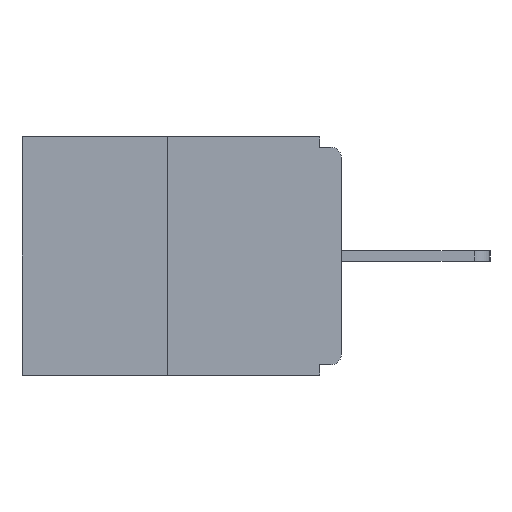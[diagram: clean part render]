
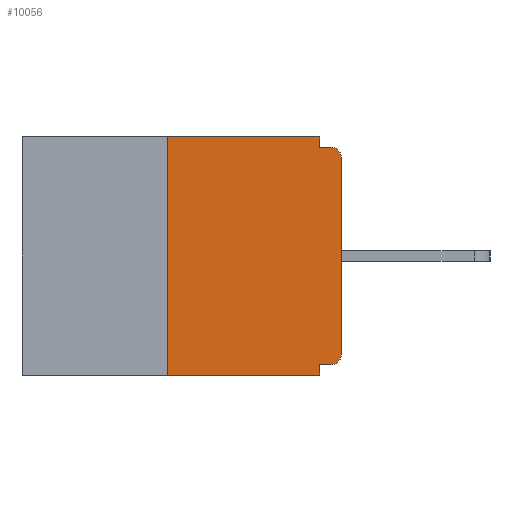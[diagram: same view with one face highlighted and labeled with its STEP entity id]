
A CAD part, left-side view. The second image highlights one B-rep face of the part: STEP entity #10056.
In plain terms, the highlighted planar face has unit normal (-1, 0, 0).
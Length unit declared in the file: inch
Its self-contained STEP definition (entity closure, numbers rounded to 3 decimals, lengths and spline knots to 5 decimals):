
#60 = PLANE ( 'NONE',  #2850 ) ;
#109 = ORIENTED_EDGE ( 'NONE', *, *, #1626, .F. ) ;
#178 = EDGE_LOOP ( 'NONE', ( #8929, #3693, #7737, #2448, #1914, #5647, #10273, #12927, #10424, #109 ) ) ;
#331 = EDGE_CURVE ( 'NONE', #2120, #7161, #4536, .T. ) ;
#432 = LINE ( 'NONE', #6537, #1661 ) ;
#465 = VECTOR ( 'NONE', #6423, 39.37008 ) ;
#608 = VERTEX_POINT ( 'NONE', #2188 ) ;
#852 = DIRECTION ( 'NONE',  ( 0., 0., -1. ) ) ;
#990 = CARTESIAN_POINT ( 'NONE',  ( 0., 0.25, 0. ) ) ;
#1165 = CARTESIAN_POINT ( 'NONE',  ( 0., 0.031, -0.343 ) ) ;
#1224 = VERTEX_POINT ( 'NONE', #3137 ) ;
#1465 = CIRCLE ( 'NONE', #7824, 0.015 ) ;
#1480 = CARTESIAN_POINT ( 'NONE',  ( 0., 0.015, -0.015 ) ) ;
#1555 = CARTESIAN_POINT ( 'NONE',  ( 0., 0., -0.03 ) ) ;
#1626 = EDGE_CURVE ( 'NONE', #608, #5950, #11056, .T. ) ;
#1661 = VECTOR ( 'NONE', #6467, 39.37008 ) ;
#1708 = CARTESIAN_POINT ( 'NONE',  ( 0., 0.015, -0.03 ) ) ;
#1912 = CARTESIAN_POINT ( 'NONE',  ( 0., 0.031, -0.343 ) ) ;
#1914 = ORIENTED_EDGE ( 'NONE', *, *, #2885, .F. ) ;
#2120 = VERTEX_POINT ( 'NONE', #7968 ) ;
#2123 = VECTOR ( 'NONE', #10434, 39.37008 ) ;
#2188 = CARTESIAN_POINT ( 'NONE',  ( 0., 0.031, 0. ) ) ;
#2448 = ORIENTED_EDGE ( 'NONE', *, *, #10078, .F. ) ;
#2670 = EDGE_CURVE ( 'NONE', #10574, #12998, #432, .T. ) ;
#2810 = DIRECTION ( 'NONE',  ( -1., 0., 0. ) ) ;
#2850 = AXIS2_PLACEMENT_3D ( 'NONE', #4093, #8013, #12083 ) ;
#2885 = EDGE_CURVE ( 'NONE', #8611, #1224, #9465, .T. ) ;
#3069 = VECTOR ( 'NONE', #5121, 39.37008 ) ;
#3137 = CARTESIAN_POINT ( 'NONE',  ( 0., 0.031, -0.328 ) ) ;
#3693 = ORIENTED_EDGE ( 'NONE', *, *, #331, .F. ) ;
#3804 = VECTOR ( 'NONE', #7784, 39.37008 ) ;
#4093 = CARTESIAN_POINT ( 'NONE',  ( 0., 0.46, 0. ) ) ;
#4132 = DIRECTION ( 'NONE',  ( 0., 1., 0. ) ) ;
#4360 = CARTESIAN_POINT ( 'NONE',  ( 0., 0.46, 0. ) ) ;
#4429 = LINE ( 'NONE', #4360, #465 ) ;
#4536 = LINE ( 'NONE', #11725, #3804 ) ;
#4790 = VERTEX_POINT ( 'NONE', #1912 ) ;
#5121 = DIRECTION ( 'NONE',  ( 0., 0., -1. ) ) ;
#5245 = EDGE_CURVE ( 'NONE', #12998, #9589, #1465, .T. ) ;
#5251 = CARTESIAN_POINT ( 'NONE',  ( 0., 0., -0.328 ) ) ;
#5427 = CARTESIAN_POINT ( 'NONE',  ( 0., 0., -0.015 ) ) ;
#5647 = ORIENTED_EDGE ( 'NONE', *, *, #12680, .T. ) ;
#5749 = DIRECTION ( 'NONE',  ( -1., 0., 0. ) ) ;
#5808 = CARTESIAN_POINT ( 'NONE',  ( 0., 0.015, -0.313 ) ) ;
#5950 = VERTEX_POINT ( 'NONE', #10644 ) ;
#6162 = EDGE_CURVE ( 'NONE', #5950, #9589, #8215, .T. ) ;
#6244 = VECTOR ( 'NONE', #11150, 39.37008 ) ;
#6365 = VECTOR ( 'NONE', #9177, 39.37008 ) ;
#6423 = DIRECTION ( 'NONE',  ( 0., -1., 0. ) ) ;
#6467 = DIRECTION ( 'NONE',  ( 0., 0., 1. ) ) ;
#6537 = CARTESIAN_POINT ( 'NONE',  ( 0., 0., 0. ) ) ;
#6703 = AXIS2_PLACEMENT_3D ( 'NONE', #5808, #2810, #10951 ) ;
#6748 = EDGE_CURVE ( 'NONE', #2120, #4790, #12362, .T. ) ;
#7029 = LINE ( 'NONE', #1165, #6244 ) ;
#7161 = VERTEX_POINT ( 'NONE', #990 ) ;
#7297 = CARTESIAN_POINT ( 'NONE',  ( 0., 0.46, -0.343 ) ) ;
#7299 = EDGE_CURVE ( 'NONE', #7161, #608, #4429, .T. ) ;
#7737 = ORIENTED_EDGE ( 'NONE', *, *, #6748, .T. ) ;
#7784 = DIRECTION ( 'NONE',  ( 0., 0., 1. ) ) ;
#7824 = AXIS2_PLACEMENT_3D ( 'NONE', #1708, #5749, #852 ) ;
#7968 = CARTESIAN_POINT ( 'NONE',  ( 0., 0.25, -0.343 ) ) ;
#8013 = DIRECTION ( 'NONE',  ( 1., 0., 0. ) ) ;
#8017 = VECTOR ( 'NONE', #4132, 39.37008 ) ;
#8183 = CARTESIAN_POINT ( 'NONE',  ( 0., 0., -0.313 ) ) ;
#8215 = LINE ( 'NONE', #5427, #6365 ) ;
#8611 = VERTEX_POINT ( 'NONE', #9502 ) ;
#8929 = ORIENTED_EDGE ( 'NONE', *, *, #7299, .F. ) ;
#9177 = DIRECTION ( 'NONE',  ( 0., -1., 0. ) ) ;
#9228 = FACE_OUTER_BOUND ( 'NONE', #178, .T. ) ;
#9415 = CIRCLE ( 'NONE', #6703, 0.015 ) ;
#9465 = LINE ( 'NONE', #5251, #8017 ) ;
#9502 = CARTESIAN_POINT ( 'NONE',  ( 0., 0.015, -0.328 ) ) ;
#9589 = VERTEX_POINT ( 'NONE', #1480 ) ;
#10056 = ADVANCED_FACE ( 'NONE', ( #9228 ), #60, .F. ) ;
#10078 = EDGE_CURVE ( 'NONE', #1224, #4790, #7029, .T. ) ;
#10273 = ORIENTED_EDGE ( 'NONE', *, *, #2670, .T. ) ;
#10424 = ORIENTED_EDGE ( 'NONE', *, *, #6162, .F. ) ;
#10434 = DIRECTION ( 'NONE',  ( 0., -1., 0. ) ) ;
#10574 = VERTEX_POINT ( 'NONE', #8183 ) ;
#10644 = CARTESIAN_POINT ( 'NONE',  ( 0., 0.031, -0.015 ) ) ;
#10951 = DIRECTION ( 'NONE',  ( 0., 0., -1. ) ) ;
#11056 = LINE ( 'NONE', #12182, #3069 ) ;
#11150 = DIRECTION ( 'NONE',  ( 0., 0., -1. ) ) ;
#11725 = CARTESIAN_POINT ( 'NONE',  ( 0., 0.25, 0. ) ) ;
#12083 = DIRECTION ( 'NONE',  ( 0., 0., -1. ) ) ;
#12182 = CARTESIAN_POINT ( 'NONE',  ( 0., 0.031, 0. ) ) ;
#12362 = LINE ( 'NONE', #7297, #2123 ) ;
#12680 = EDGE_CURVE ( 'NONE', #8611, #10574, #9415, .T. ) ;
#12927 = ORIENTED_EDGE ( 'NONE', *, *, #5245, .T. ) ;
#12998 = VERTEX_POINT ( 'NONE', #1555 ) ;
